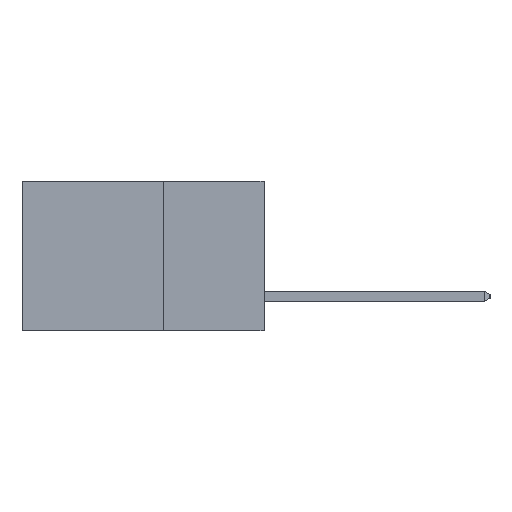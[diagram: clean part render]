
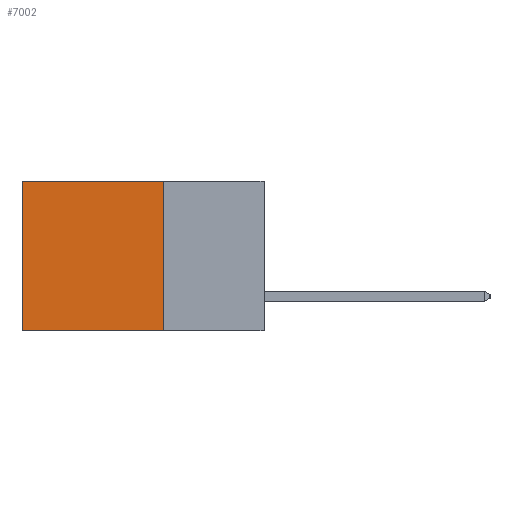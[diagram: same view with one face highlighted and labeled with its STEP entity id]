
A CAD part, left-side view. The second image highlights one B-rep face of the part: STEP entity #7002.
In plain terms, the highlighted planar face has unit normal (-1, 0, 0).
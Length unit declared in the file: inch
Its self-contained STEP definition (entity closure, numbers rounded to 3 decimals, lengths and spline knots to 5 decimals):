
#1011 = VERTEX_POINT ( 'NONE', #3356 ) ;
#1766 = FACE_OUTER_BOUND ( 'NONE', #3556, .T. ) ;
#1922 = ORIENTED_EDGE ( 'NONE', *, *, #7810, .F. ) ;
#1974 = ORIENTED_EDGE ( 'NONE', *, *, #12790, .T. ) ;
#2047 = LINE ( 'NONE', #13602, #8553 ) ;
#2051 = EDGE_CURVE ( 'NONE', #1011, #2860, #13682, .T. ) ;
#2139 = CARTESIAN_POINT ( 'NONE',  ( 0.298, 0.6, 0. ) ) ;
#2287 = DIRECTION ( 'NONE',  ( 0., 0., -1. ) ) ;
#2350 = CARTESIAN_POINT ( 'NONE',  ( 0.298, 0.6, 0. ) ) ;
#2860 = VERTEX_POINT ( 'NONE', #2139 ) ;
#3356 = CARTESIAN_POINT ( 'NONE',  ( 0.298, 0.25, 0. ) ) ;
#3556 = EDGE_LOOP ( 'NONE', ( #1974, #1922, #9075, #14455 ) ) ;
#3689 = LINE ( 'NONE', #2350, #6956 ) ;
#5760 = CARTESIAN_POINT ( 'NONE',  ( 0.298, 0.25, -0.37 ) ) ;
#6098 = CARTESIAN_POINT ( 'NONE',  ( 0.298, 0.25, -0.37 ) ) ;
#6118 = DIRECTION ( 'NONE',  ( 0., 0., -1. ) ) ;
#6209 = DIRECTION ( 'NONE',  ( 1., 0., 0. ) ) ;
#6933 = DIRECTION ( 'NONE',  ( 0., 0., -1. ) ) ;
#6956 = VECTOR ( 'NONE', #2287, 39.37008 ) ;
#7002 = ADVANCED_FACE ( 'NONE', ( #1766 ), #7470, .F. ) ;
#7028 = VERTEX_POINT ( 'NONE', #8406 ) ;
#7470 = PLANE ( 'NONE',  #12902 ) ;
#7810 = EDGE_CURVE ( 'NONE', #16648, #7028, #12743, .T. ) ;
#8406 = CARTESIAN_POINT ( 'NONE',  ( 0.298, 0.6, -0.37 ) ) ;
#8441 = CARTESIAN_POINT ( 'NONE',  ( 0.298, 0.25, 0. ) ) ;
#8553 = VECTOR ( 'NONE', #6933, 39.37008 ) ;
#8694 = VECTOR ( 'NONE', #10109, 39.37008 ) ;
#9075 = ORIENTED_EDGE ( 'NONE', *, *, #13917, .F. ) ;
#9999 = CARTESIAN_POINT ( 'NONE',  ( 0.298, 0.25, 0. ) ) ;
#10106 = VECTOR ( 'NONE', #11264, 39.37008 ) ;
#10109 = DIRECTION ( 'NONE',  ( 0., 1., 0. ) ) ;
#11264 = DIRECTION ( 'NONE',  ( 0., 1., 0. ) ) ;
#12743 = LINE ( 'NONE', #6098, #8694 ) ;
#12790 = EDGE_CURVE ( 'NONE', #2860, #7028, #3689, .T. ) ;
#12902 = AXIS2_PLACEMENT_3D ( 'NONE', #8441, #6209, #6118 ) ;
#13602 = CARTESIAN_POINT ( 'NONE',  ( 0.298, 0.25, 0. ) ) ;
#13682 = LINE ( 'NONE', #9999, #10106 ) ;
#13917 = EDGE_CURVE ( 'NONE', #1011, #16648, #2047, .T. ) ;
#14455 = ORIENTED_EDGE ( 'NONE', *, *, #2051, .T. ) ;
#16648 = VERTEX_POINT ( 'NONE', #5760 ) ;
